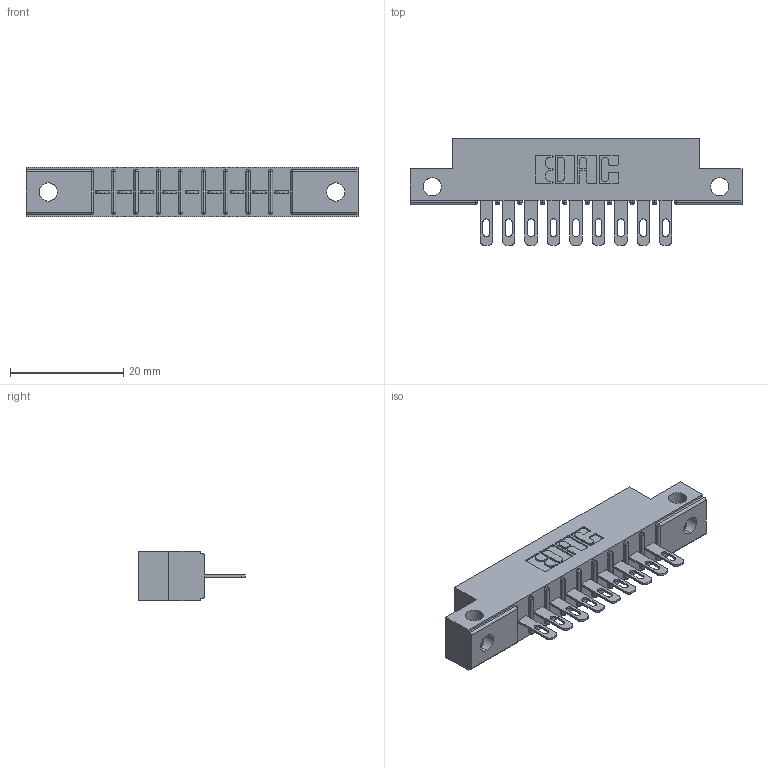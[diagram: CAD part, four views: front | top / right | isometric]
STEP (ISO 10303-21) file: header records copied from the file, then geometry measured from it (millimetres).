
FILE_DESCRIPTION (( 'STEP AP203' ), '1' );
FILE_NAME ('316-009-400-112.STEP', '2020-09-22T14:50:24', ( '' ), ( '' ), 'SwSTEP 2.0', 'SolidWorks 2020', '' );
FILE_SCHEMA (( 'CONFIG_CONTROL_DESIGN' ));
Length unit declared in the file: inch
Products named in the file (3): 306 Part_.128 Dia; 316-009-400-112; 306-290-001_100
Assembly tree (10 placements, depth 2):
  316-009-400-112
    306 Part_.128 Dia
    306-290-001_100  x9
Bounding box: 58.67 x 18.87 x 8.71 mm (x, y, z)
Volume: 3852.9 mm3; surface area: 5365.8 mm2
Topology: 10 solids, 10 shells, 812 faces, 2287 edges, 1470 vertices
Faces by surface type: plane 518, cylinder 258, sphere 36
Entity records: 13238 total; most frequent: CARTESIAN_POINT 2266, ORIENTED_EDGE 2198, DIRECTION 2177, EDGE_CURVE 1099, LINE 823, VECTOR 823, VERTEX_POINT 702, AXIS2_PLACEMENT_3D 677
